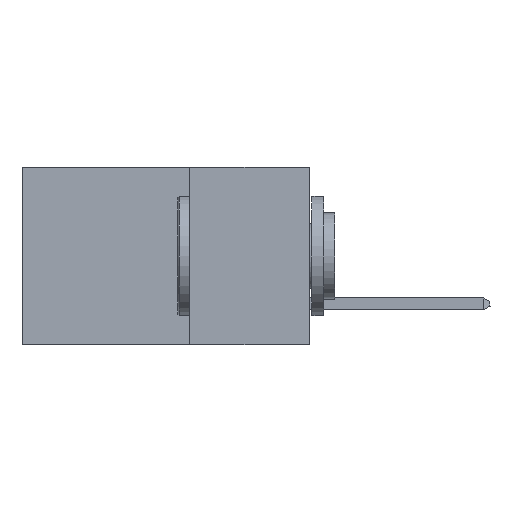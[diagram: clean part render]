
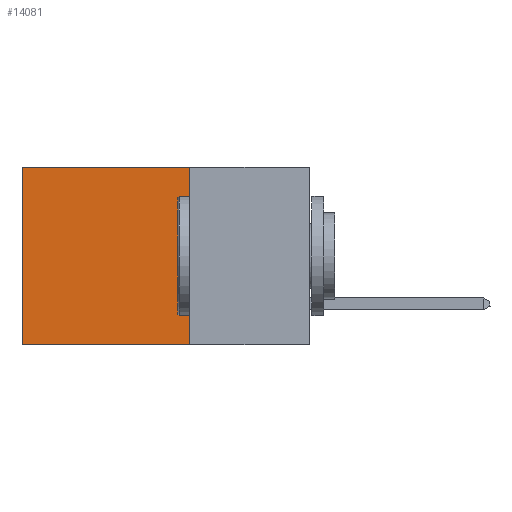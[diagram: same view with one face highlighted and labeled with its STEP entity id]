
A CAD part, left-side view. The second image highlights one B-rep face of the part: STEP entity #14081.
In plain terms, the highlighted planar face has unit normal (-1, 0, 0).
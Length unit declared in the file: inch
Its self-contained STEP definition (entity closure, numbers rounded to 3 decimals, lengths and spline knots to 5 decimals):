
#808 = ORIENTED_EDGE ( 'NONE', *, *, #14107, .T. ) ;
#1319 = ORIENTED_EDGE ( 'NONE', *, *, #16980, .T. ) ;
#1721 = VECTOR ( 'NONE', #24363, 39.37008 ) ;
#2117 = DIRECTION ( 'NONE',  ( 0., 0., -1. ) ) ;
#2645 = CARTESIAN_POINT ( 'NONE',  ( 0.2875, 0.25, -0.37 ) ) ;
#4342 = DIRECTION ( 'NONE',  ( 0., 0., -1. ) ) ;
#5115 = VERTEX_POINT ( 'NONE', #6194 ) ;
#6194 = CARTESIAN_POINT ( 'NONE',  ( 0.2875, 0.25, 0. ) ) ;
#6318 = CARTESIAN_POINT ( 'NONE',  ( 0.2875, 0.25, 0. ) ) ;
#6396 = VERTEX_POINT ( 'NONE', #9116 ) ;
#7477 = EDGE_CURVE ( 'NONE', #5115, #22144, #11683, .T. ) ;
#7888 = LINE ( 'NONE', #6318, #1721 ) ;
#8179 = VECTOR ( 'NONE', #21329, 39.37008 ) ;
#8853 = LINE ( 'NONE', #11339, #8179 ) ;
#9116 = CARTESIAN_POINT ( 'NONE',  ( 0.2875, 0.6, -0.37 ) ) ;
#9767 = VECTOR ( 'NONE', #4342, 39.37008 ) ;
#9851 = CARTESIAN_POINT ( 'NONE',  ( 0.2875, 0.6, 0. ) ) ;
#10346 = PLANE ( 'NONE',  #21451 ) ;
#11286 = VERTEX_POINT ( 'NONE', #15804 ) ;
#11339 = CARTESIAN_POINT ( 'NONE',  ( 0.2875, 0.25, -0.37 ) ) ;
#11683 = LINE ( 'NONE', #18599, #9767 ) ;
#12024 = ORIENTED_EDGE ( 'NONE', *, *, #21670, .F. ) ;
#14081 = ADVANCED_FACE ( 'NONE', ( #23891 ), #10346, .F. ) ;
#14107 = EDGE_CURVE ( 'NONE', #5115, #11286, #7888, .T. ) ;
#14491 = DIRECTION ( 'NONE',  ( 1., 0., 0. ) ) ;
#15752 = LINE ( 'NONE', #9851, #20359 ) ;
#15804 = CARTESIAN_POINT ( 'NONE',  ( 0.2875, 0.6, 0. ) ) ;
#16980 = EDGE_CURVE ( 'NONE', #11286, #6396, #15752, .T. ) ;
#18599 = CARTESIAN_POINT ( 'NONE',  ( 0.2875, 0.25, 0. ) ) ;
#18733 = EDGE_LOOP ( 'NONE', ( #1319, #12024, #25327, #808 ) ) ;
#20359 = VECTOR ( 'NONE', #21872, 39.37008 ) ;
#21329 = DIRECTION ( 'NONE',  ( 0., 1., 0. ) ) ;
#21451 = AXIS2_PLACEMENT_3D ( 'NONE', #24290, #14491, #2117 ) ;
#21670 = EDGE_CURVE ( 'NONE', #22144, #6396, #8853, .T. ) ;
#21872 = DIRECTION ( 'NONE',  ( 0., 0., -1. ) ) ;
#22144 = VERTEX_POINT ( 'NONE', #2645 ) ;
#23891 = FACE_OUTER_BOUND ( 'NONE', #18733, .T. ) ;
#24290 = CARTESIAN_POINT ( 'NONE',  ( 0.2875, 0.25, 0. ) ) ;
#24363 = DIRECTION ( 'NONE',  ( 0., 1., 0. ) ) ;
#25327 = ORIENTED_EDGE ( 'NONE', *, *, #7477, .F. ) ;
